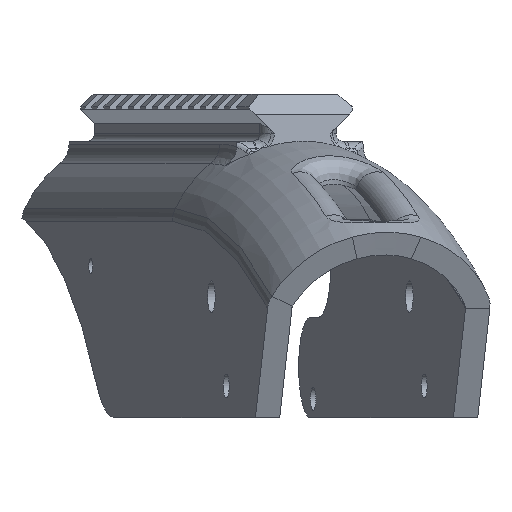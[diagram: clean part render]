
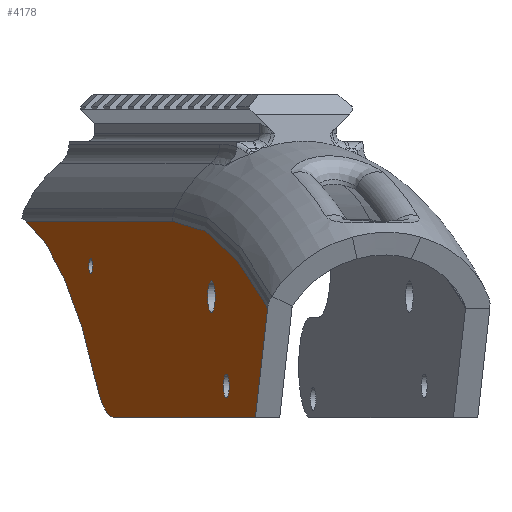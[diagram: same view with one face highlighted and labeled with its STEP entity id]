
A CAD part, left-side view. The second image highlights one B-rep face of the part: STEP entity #4178.
In plain terms, the highlighted planar face has unit normal (-0.241, 0.971, 0).
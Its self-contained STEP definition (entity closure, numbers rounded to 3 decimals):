
#57=PLANE('',#4433);
#187=FACE_BOUND('',#1460,.T.);
#188=FACE_BOUND('',#1461,.T.);
#189=FACE_BOUND('',#1462,.T.);
#190=FACE_BOUND('',#1463,.T.);
#219=LINE('',#6207,#617);
#224=LINE('',#6231,#622);
#225=LINE('',#6235,#623);
#617=VECTOR('',#4733,116.808);
#622=VECTOR('',#4756,24.133);
#623=VECTOR('',#4759,121.456);
#1460=EDGE_LOOP('',(#2941));
#1461=EDGE_LOOP('',(#2942,#2943,#2944,#2945,#2946,#2947));
#1462=EDGE_LOOP('',(#2948));
#1463=EDGE_LOOP('',(#2949));
#1717=CIRCLE('',#4434,1.55);
#1718=CIRCLE('',#4435,188.817);
#1719=CIRCLE('',#4436,105.792);
#1720=CIRCLE('',#4437,20.);
#1721=CIRCLE('',#4438,3.16);
#1722=CIRCLE('',#4439,2.375);
#1830=VERTEX_POINT('',#6203);
#1832=VERTEX_POINT('',#6206);
#1841=VERTEX_POINT('',#6228);
#1842=VERTEX_POINT('',#6230);
#1843=VERTEX_POINT('',#6232);
#1844=VERTEX_POINT('',#6234);
#1845=VERTEX_POINT('',#6236);
#1846=VERTEX_POINT('',#6239);
#1847=VERTEX_POINT('',#6241);
#2266=EDGE_CURVE('',#1832,#1830,#219,.T.);
#2277=EDGE_CURVE('',#1841,#1841,#1717,.F.);
#2278=EDGE_CURVE('',#1842,#1830,#224,.T.);
#2279=EDGE_CURVE('',#1843,#1842,#1718,.T.);
#2280=EDGE_CURVE('',#1844,#1843,#225,.T.);
#2281=EDGE_CURVE('',#1844,#1845,#1719,.T.);
#2282=EDGE_CURVE('',#1832,#1845,#1720,.T.);
#2283=EDGE_CURVE('',#1846,#1846,#1721,.F.);
#2284=EDGE_CURVE('',#1847,#1847,#1722,.F.);
#2941=ORIENTED_EDGE('',*,*,#2277,.F.);
#2942=ORIENTED_EDGE('',*,*,#2266,.T.);
#2943=ORIENTED_EDGE('',*,*,#2278,.F.);
#2944=ORIENTED_EDGE('',*,*,#2279,.F.);
#2945=ORIENTED_EDGE('',*,*,#2280,.F.);
#2946=ORIENTED_EDGE('',*,*,#2281,.T.);
#2947=ORIENTED_EDGE('',*,*,#2282,.F.);
#2948=ORIENTED_EDGE('',*,*,#2283,.F.);
#2949=ORIENTED_EDGE('',*,*,#2284,.F.);
#4178=ADVANCED_FACE('',(#187,#188,#189,#190),#57,.F.);
#4433=AXIS2_PLACEMENT_3D('',#6227,#4752,#4753);
#4434=AXIS2_PLACEMENT_3D('',#6229,#4754,#4755);
#4435=AXIS2_PLACEMENT_3D('',#6233,#4757,#4758);
#4436=AXIS2_PLACEMENT_3D('',#6237,#4760,#4761);
#4437=AXIS2_PLACEMENT_3D('',#6238,#4762,#4763);
#4438=AXIS2_PLACEMENT_3D('',#6240,#4764,#4765);
#4439=AXIS2_PLACEMENT_3D('',#6242,#4766,#4767);
#4733=DIRECTION('',(-0.971,-0.241,0.));
#4752=DIRECTION('center_axis',(0.241,-0.971,0.));
#4753=DIRECTION('ref_axis',(-0.97,-0.24,-0.048));
#4754=DIRECTION('center_axis',(0.241,-0.971,0.));
#4755=DIRECTION('ref_axis',(0.,0.,-1.));
#4756=DIRECTION('',(0.406,0.101,-0.908));
#4757=DIRECTION('center_axis',(0.241,-0.971,0.));
#4758=DIRECTION('ref_axis',(0.,0.,-1.));
#4759=DIRECTION('',(-0.971,-0.241,0.));
#4760=DIRECTION('center_axis',(0.241,-0.971,0.));
#4761=DIRECTION('ref_axis',(-0.78,-0.193,0.595));
#4762=DIRECTION('center_axis',(0.241,-0.971,0.));
#4763=DIRECTION('ref_axis',(0.392,0.097,-0.915));
#4764=DIRECTION('center_axis',(0.241,-0.971,0.));
#4765=DIRECTION('ref_axis',(0.,0.,-1.));
#4766=DIRECTION('center_axis',(0.241,-0.971,0.));
#4767=DIRECTION('ref_axis',(0.,0.,-1.));
#6203=CARTESIAN_POINT('',(-587.352,-71.72,46.392));
#6206=CARTESIAN_POINT('',(-473.974,-43.619,46.392));
#6207=CARTESIAN_POINT('',(-493.397,-48.433,46.392));
#6227=CARTESIAN_POINT('Origin',(-527.481,-56.881,62.29));
#6228=CARTESIAN_POINT('',(-453.213,-38.474,76.68));
#6229=CARTESIAN_POINT('Origin',(-454.717,-38.847,76.68));
#6230=CARTESIAN_POINT('',(-597.144,-74.147,68.315));
#6231=CARTESIAN_POINT('',(-590.215,-72.429,52.802));
#6232=CARTESIAN_POINT('',(-520.526,-55.157,85.607));
#6233=CARTESIAN_POINT('Origin',(-520.526,-55.157,-103.21));
#6234=CARTESIAN_POINT('',(-402.636,-25.939,85.607));
#6235=CARTESIAN_POINT('',(-499.169,-49.864,85.607));
#6236=CARTESIAN_POINT('',(-459.632,-40.065,52.913));
#6237=CARTESIAN_POINT('Origin',(-383.769,-21.263,-18.384));
#6238=CARTESIAN_POINT('Origin',(-473.974,-43.619,66.392));
#6239=CARTESIAN_POINT('',(-548.81,-62.167,70.562));
#6240=CARTESIAN_POINT('Origin',(-551.877,-62.927,70.562));
#6241=CARTESIAN_POINT('',(-561.559,-65.327,52.75));
#6242=CARTESIAN_POINT('Origin',(-563.865,-65.898,52.75));
